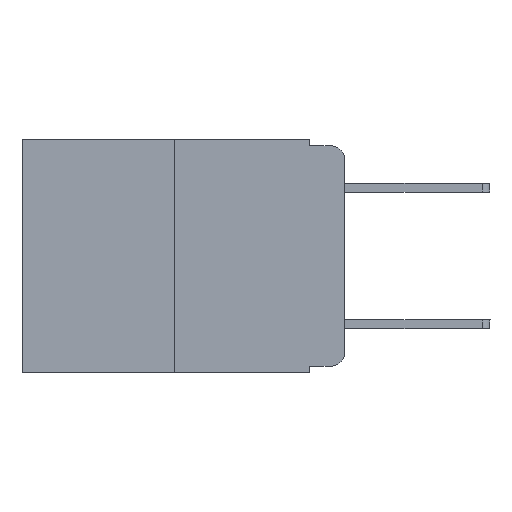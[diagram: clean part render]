
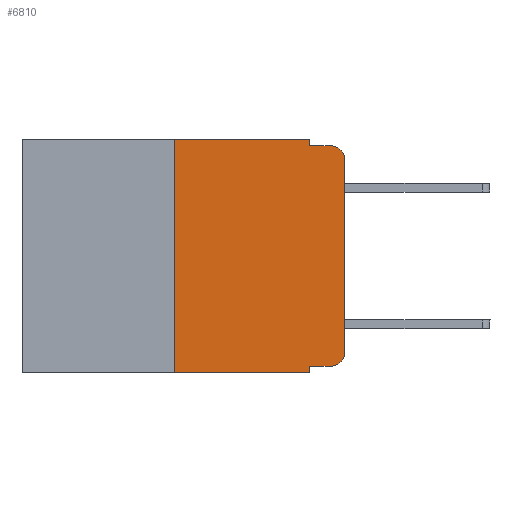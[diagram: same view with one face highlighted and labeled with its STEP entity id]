
A CAD part, left-side view. The second image highlights one B-rep face of the part: STEP entity #6810.
In plain terms, the highlighted planar face has unit normal (-1, 0, 0).
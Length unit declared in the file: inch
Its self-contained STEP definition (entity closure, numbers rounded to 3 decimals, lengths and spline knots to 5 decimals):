
#55 = ORIENTED_EDGE ( 'NONE', *, *, #17770, .F. ) ;
#863 = AXIS2_PLACEMENT_3D ( 'NONE', #8435, #2393, #8506 ) ;
#1531 = DIRECTION ( 'NONE',  ( -1., 0., 0. ) ) ;
#2247 = VERTEX_POINT ( 'NONE', #20072 ) ;
#2257 = CARTESIAN_POINT ( 'NONE',  ( 0., 0.02, -0.01 ) ) ;
#2393 = DIRECTION ( 'NONE',  ( 1., 0., 0. ) ) ;
#2986 = CARTESIAN_POINT ( 'NONE',  ( 0., 0.473, -0.343 ) ) ;
#3239 = FACE_OUTER_BOUND ( 'NONE', #10696, .T. ) ;
#3311 = CARTESIAN_POINT ( 'NONE',  ( 0., 0.051, -0.333 ) ) ;
#3343 = EDGE_CURVE ( 'NONE', #11466, #12518, #3783, .T. ) ;
#3500 = CARTESIAN_POINT ( 'NONE',  ( 0., 0.051, -0.343 ) ) ;
#3679 = VECTOR ( 'NONE', #4221, 39.37008 ) ;
#3783 = CIRCLE ( 'NONE', #11364, 0.02 ) ;
#4221 = DIRECTION ( 'NONE',  ( 0., 0., -1. ) ) ;
#4380 = CARTESIAN_POINT ( 'NONE',  ( 0., 0.02, -0.03 ) ) ;
#4814 = LINE ( 'NONE', #19520, #12845 ) ;
#4869 = EDGE_CURVE ( 'NONE', #18945, #2247, #6622, .T. ) ;
#5254 = VECTOR ( 'NONE', #18590, 39.37008 ) ;
#5395 = LINE ( 'NONE', #7909, #11726 ) ;
#5629 = LINE ( 'NONE', #3311, #15864 ) ;
#6097 = CARTESIAN_POINT ( 'NONE',  ( 0., 0.25, 0. ) ) ;
#6622 = LINE ( 'NONE', #10023, #18060 ) ;
#6779 = DIRECTION ( 'NONE',  ( 0., 0., -1. ) ) ;
#6810 = ADVANCED_FACE ( 'NONE', ( #3239 ), #17734, .F. ) ;
#6812 = ORIENTED_EDGE ( 'NONE', *, *, #10592, .T. ) ;
#7231 = DIRECTION ( 'NONE',  ( 0., 0., 1. ) ) ;
#7373 = VERTEX_POINT ( 'NONE', #3500 ) ;
#7646 = EDGE_CURVE ( 'NONE', #13354, #11466, #5629, .T. ) ;
#7909 = CARTESIAN_POINT ( 'NONE',  ( 0., 0.051, -0.01 ) ) ;
#8168 = DIRECTION ( 'NONE',  ( -1., 0., 0. ) ) ;
#8213 = ORIENTED_EDGE ( 'NONE', *, *, #16251, .F. ) ;
#8278 = LINE ( 'NONE', #2986, #8513 ) ;
#8435 = CARTESIAN_POINT ( 'NONE',  ( 0., 0.473, 0. ) ) ;
#8506 = DIRECTION ( 'NONE',  ( 0., 0., -1. ) ) ;
#8513 = VECTOR ( 'NONE', #13844, 39.37008 ) ;
#8897 = ORIENTED_EDGE ( 'NONE', *, *, #15353, .T. ) ;
#9099 = CIRCLE ( 'NONE', #17747, 0.02 ) ;
#10023 = CARTESIAN_POINT ( 'NONE',  ( 0., 0.473, 0. ) ) ;
#10592 = EDGE_CURVE ( 'NONE', #12518, #11476, #4814, .T. ) ;
#10696 = EDGE_LOOP ( 'NONE', ( #6812, #8897, #8213, #14833, #12203, #14913, #10750, #55, #19228, #12437 ) ) ;
#10750 = ORIENTED_EDGE ( 'NONE', *, *, #18241, .T. ) ;
#10983 = CARTESIAN_POINT ( 'NONE',  ( 0., 0.25, 0. ) ) ;
#11320 = DIRECTION ( 'NONE',  ( 0., -1., 0. ) ) ;
#11364 = AXIS2_PLACEMENT_3D ( 'NONE', #11366, #8168, #6779 ) ;
#11366 = CARTESIAN_POINT ( 'NONE',  ( 0., 0.02, -0.313 ) ) ;
#11466 = VERTEX_POINT ( 'NONE', #15771 ) ;
#11476 = VERTEX_POINT ( 'NONE', #15510 ) ;
#11726 = VECTOR ( 'NONE', #11320, 39.37008 ) ;
#12044 = DIRECTION ( 'NONE',  ( 0., 0., -1. ) ) ;
#12083 = CARTESIAN_POINT ( 'NONE',  ( 0., 0.051, -0.333 ) ) ;
#12203 = ORIENTED_EDGE ( 'NONE', *, *, #4869, .F. ) ;
#12437 = ORIENTED_EDGE ( 'NONE', *, *, #3343, .T. ) ;
#12518 = VERTEX_POINT ( 'NONE', #20073 ) ;
#12845 = VECTOR ( 'NONE', #7231, 39.37008 ) ;
#13130 = DIRECTION ( 'NONE',  ( 0., -1., 0. ) ) ;
#13354 = VERTEX_POINT ( 'NONE', #12083 ) ;
#13362 = VECTOR ( 'NONE', #12044, 39.37008 ) ;
#13553 = CARTESIAN_POINT ( 'NONE',  ( 0., 0.051, 0. ) ) ;
#13680 = DIRECTION ( 'NONE',  ( 0., -1., 0. ) ) ;
#13800 = CARTESIAN_POINT ( 'NONE',  ( 0., 0.25, -0.343 ) ) ;
#13844 = DIRECTION ( 'NONE',  ( 0., -1., 0. ) ) ;
#14833 = ORIENTED_EDGE ( 'NONE', *, *, #16987, .F. ) ;
#14913 = ORIENTED_EDGE ( 'NONE', *, *, #19961, .F. ) ;
#15353 = EDGE_CURVE ( 'NONE', #11476, #19521, #9099, .T. ) ;
#15510 = CARTESIAN_POINT ( 'NONE',  ( 0., 0., -0.03 ) ) ;
#15771 = CARTESIAN_POINT ( 'NONE',  ( 0., 0.02, -0.333 ) ) ;
#15864 = VECTOR ( 'NONE', #13680, 39.37008 ) ;
#16081 = LINE ( 'NONE', #13553, #3679 ) ;
#16251 = EDGE_CURVE ( 'NONE', #18302, #19521, #5395, .T. ) ;
#16775 = CARTESIAN_POINT ( 'NONE',  ( 0., 0.051, -0.01 ) ) ;
#16901 = DIRECTION ( 'NONE',  ( 0., 0., -1. ) ) ;
#16987 = EDGE_CURVE ( 'NONE', #2247, #18302, #16081, .T. ) ;
#17734 = PLANE ( 'NONE',  #863 ) ;
#17747 = AXIS2_PLACEMENT_3D ( 'NONE', #4380, #1531, #16901 ) ;
#17770 = EDGE_CURVE ( 'NONE', #13354, #7373, #19649, .T. ) ;
#18060 = VECTOR ( 'NONE', #13130, 39.37008 ) ;
#18241 = EDGE_CURVE ( 'NONE', #19290, #7373, #8278, .T. ) ;
#18302 = VERTEX_POINT ( 'NONE', #16775 ) ;
#18412 = CARTESIAN_POINT ( 'NONE',  ( 0., 0.051, 0. ) ) ;
#18590 = DIRECTION ( 'NONE',  ( 0., 0., 1. ) ) ;
#18945 = VERTEX_POINT ( 'NONE', #10983 ) ;
#19228 = ORIENTED_EDGE ( 'NONE', *, *, #7646, .T. ) ;
#19290 = VERTEX_POINT ( 'NONE', #13800 ) ;
#19520 = CARTESIAN_POINT ( 'NONE',  ( 0., 0., 0. ) ) ;
#19521 = VERTEX_POINT ( 'NONE', #2257 ) ;
#19578 = LINE ( 'NONE', #6097, #5254 ) ;
#19649 = LINE ( 'NONE', #18412, #13362 ) ;
#19961 = EDGE_CURVE ( 'NONE', #19290, #18945, #19578, .T. ) ;
#20072 = CARTESIAN_POINT ( 'NONE',  ( 0., 0.051, 0. ) ) ;
#20073 = CARTESIAN_POINT ( 'NONE',  ( 0., 0., -0.313 ) ) ;
